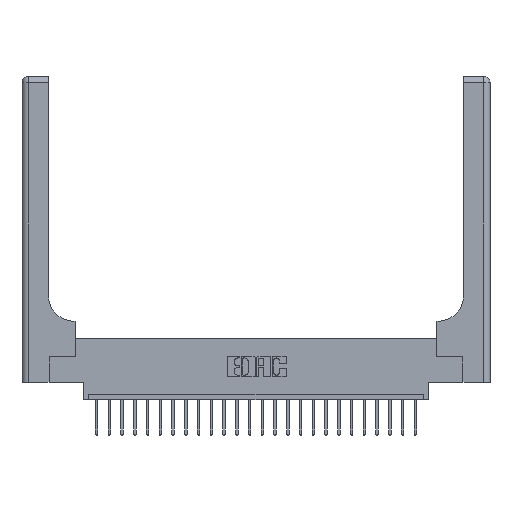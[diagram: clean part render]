
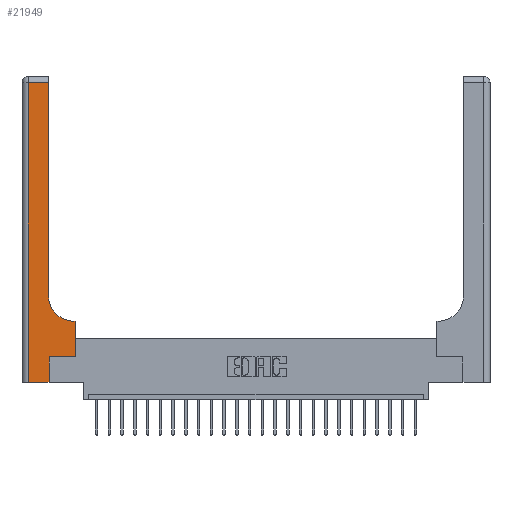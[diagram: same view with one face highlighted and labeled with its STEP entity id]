
A CAD part, top view. The second image highlights one B-rep face of the part: STEP entity #21949.
In plain terms, the highlighted planar face has unit normal (0, 0, 1).
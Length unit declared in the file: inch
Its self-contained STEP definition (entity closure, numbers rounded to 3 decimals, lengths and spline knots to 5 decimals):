
#29 = VERTEX_POINT ( 'NONE', #1958 ) ;
#78 = ORIENTED_EDGE ( 'NONE', *, *, #22419, .T. ) ;
#503 = VECTOR ( 'NONE', #12025, 39.37008 ) ;
#687 = EDGE_CURVE ( 'NONE', #19744, #5479, #19206, .T. ) ;
#1789 = VERTEX_POINT ( 'NONE', #6967 ) ;
#1822 = VECTOR ( 'NONE', #19074, 39.37008 ) ;
#1958 = CARTESIAN_POINT ( 'NONE',  ( 0.26, 0.85, 0.37 ) ) ;
#2131 = PLANE ( 'NONE',  #9423 ) ;
#2134 = ORIENTED_EDGE ( 'NONE', *, *, #12372, .T. ) ;
#2358 = DIRECTION ( 'NONE',  ( -1., 0., 0. ) ) ;
#2687 = LINE ( 'NONE', #3101, #16686 ) ;
#2810 = CARTESIAN_POINT ( 'NONE',  ( 0.26, 0.6, 0.37 ) ) ;
#3101 = CARTESIAN_POINT ( 'NONE',  ( 0.265, 0., 0.37 ) ) ;
#3724 = VECTOR ( 'NONE', #22608, 39.37008 ) ;
#3880 = LINE ( 'NONE', #16194, #20967 ) ;
#3914 = ORIENTED_EDGE ( 'NONE', *, *, #16626, .T. ) ;
#4990 = ORIENTED_EDGE ( 'NONE', *, *, #23531, .T. ) ;
#5018 = DIRECTION ( 'NONE',  ( 0., 1., 0. ) ) ;
#5479 = VERTEX_POINT ( 'NONE', #9870 ) ;
#5893 = CARTESIAN_POINT ( 'NONE',  ( 0., 3., 0.37 ) ) ;
#5932 = ORIENTED_EDGE ( 'NONE', *, *, #6941, .T. ) ;
#6941 = EDGE_CURVE ( 'NONE', #13509, #12369, #11440, .T. ) ;
#6967 = CARTESIAN_POINT ( 'NONE',  ( 0.26, 2.94, 0.37 ) ) ;
#7151 = VECTOR ( 'NONE', #10609, 39.37008 ) ;
#7881 = CARTESIAN_POINT ( 'NONE',  ( 0., 0., 0.37 ) ) ;
#9135 = VECTOR ( 'NONE', #23138, 39.37008 ) ;
#9423 = AXIS2_PLACEMENT_3D ( 'NONE', #5893, #13294, #2358 ) ;
#9822 = CARTESIAN_POINT ( 'NONE',  ( 0.51, 0.6, 0.37 ) ) ;
#9870 = CARTESIAN_POINT ( 'NONE',  ( 0.528, 0.6, 0.37 ) ) ;
#9955 = EDGE_CURVE ( 'NONE', #10159, #29, #20670, .T. ) ;
#9958 = LINE ( 'NONE', #16009, #9135 ) ;
#10159 = VERTEX_POINT ( 'NONE', #9822 ) ;
#10202 = LINE ( 'NONE', #2810, #503 ) ;
#10565 = DIRECTION ( 'NONE',  ( 0., 0., -1. ) ) ;
#10586 = DIRECTION ( 'NONE',  ( -1., 0., 0. ) ) ;
#10609 = DIRECTION ( 'NONE',  ( 0., -1., 0. ) ) ;
#11440 = LINE ( 'NONE', #23265, #7151 ) ;
#11539 = ORIENTED_EDGE ( 'NONE', *, *, #22897, .T. ) ;
#11853 = CARTESIAN_POINT ( 'NONE',  ( 0.528, 0.25, 0.37 ) ) ;
#12025 = DIRECTION ( 'NONE',  ( -1., 0., 0. ) ) ;
#12369 = VERTEX_POINT ( 'NONE', #22373 ) ;
#12372 = EDGE_CURVE ( 'NONE', #12369, #17194, #13975, .T. ) ;
#12488 = FACE_OUTER_BOUND ( 'NONE', #18062, .T. ) ;
#13213 = AXIS2_PLACEMENT_3D ( 'NONE', #23536, #10565, #19782 ) ;
#13294 = DIRECTION ( 'NONE',  ( 0., 0., -1. ) ) ;
#13509 = VERTEX_POINT ( 'NONE', #19317 ) ;
#13975 = LINE ( 'NONE', #7881, #3724 ) ;
#14035 = DIRECTION ( 'NONE',  ( 0., 1., 0. ) ) ;
#15938 = ORIENTED_EDGE ( 'NONE', *, *, #9955, .T. ) ;
#16009 = CARTESIAN_POINT ( 'NONE',  ( 0.265, 0.25, 0.37 ) ) ;
#16194 = CARTESIAN_POINT ( 'NONE',  ( 0., 2.94, 0.37 ) ) ;
#16626 = EDGE_CURVE ( 'NONE', #5479, #10159, #10202, .T. ) ;
#16686 = VECTOR ( 'NONE', #5018, 39.37008 ) ;
#16694 = ORIENTED_EDGE ( 'NONE', *, *, #687, .T. ) ;
#16875 = CARTESIAN_POINT ( 'NONE',  ( 0.265, 0.25, 0.37 ) ) ;
#17170 = CARTESIAN_POINT ( 'NONE',  ( 0.528, 0.25, 0.37 ) ) ;
#17194 = VERTEX_POINT ( 'NONE', #19553 ) ;
#18062 = EDGE_LOOP ( 'NONE', ( #4990, #78, #5932, #2134, #11539, #18655, #16694, #3914, #15938 ) ) ;
#18093 = LINE ( 'NONE', #20877, #1822 ) ;
#18655 = ORIENTED_EDGE ( 'NONE', *, *, #20884, .T. ) ;
#19074 = DIRECTION ( 'NONE',  ( 0., 1., 0. ) ) ;
#19206 = LINE ( 'NONE', #11853, #23246 ) ;
#19317 = CARTESIAN_POINT ( 'NONE',  ( 0.06, 2.94, 0.37 ) ) ;
#19553 = CARTESIAN_POINT ( 'NONE',  ( 0.265, 0., 0.37 ) ) ;
#19744 = VERTEX_POINT ( 'NONE', #17170 ) ;
#19782 = DIRECTION ( 'NONE',  ( 1., 0., 0. ) ) ;
#20670 = CIRCLE ( 'NONE', #13213, 0.25 ) ;
#20877 = CARTESIAN_POINT ( 'NONE',  ( 0.26, 3., 0.37 ) ) ;
#20884 = EDGE_CURVE ( 'NONE', #21933, #19744, #9958, .T. ) ;
#20967 = VECTOR ( 'NONE', #10586, 39.37008 ) ;
#21933 = VERTEX_POINT ( 'NONE', #16875 ) ;
#21949 = ADVANCED_FACE ( 'NONE', ( #12488 ), #2131, .F. ) ;
#22373 = CARTESIAN_POINT ( 'NONE',  ( 0.06, 0., 0.37 ) ) ;
#22419 = EDGE_CURVE ( 'NONE', #1789, #13509, #3880, .T. ) ;
#22608 = DIRECTION ( 'NONE',  ( 1., 0., 0. ) ) ;
#22897 = EDGE_CURVE ( 'NONE', #17194, #21933, #2687, .T. ) ;
#23138 = DIRECTION ( 'NONE',  ( 1., 0., 0. ) ) ;
#23246 = VECTOR ( 'NONE', #14035, 39.37008 ) ;
#23265 = CARTESIAN_POINT ( 'NONE',  ( 0.06, 3., 0.37 ) ) ;
#23531 = EDGE_CURVE ( 'NONE', #29, #1789, #18093, .T. ) ;
#23536 = CARTESIAN_POINT ( 'NONE',  ( 0.51, 0.85, 0.37 ) ) ;
